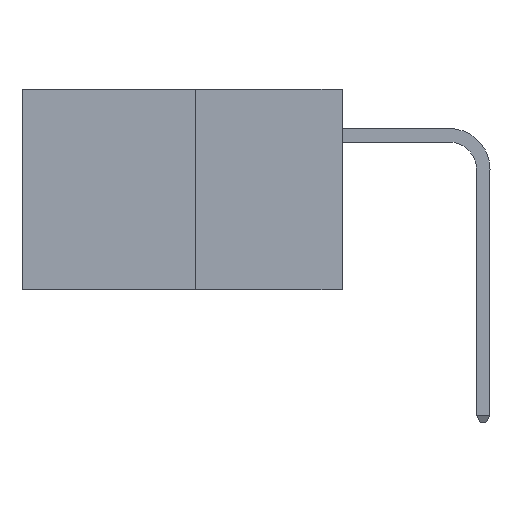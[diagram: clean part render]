
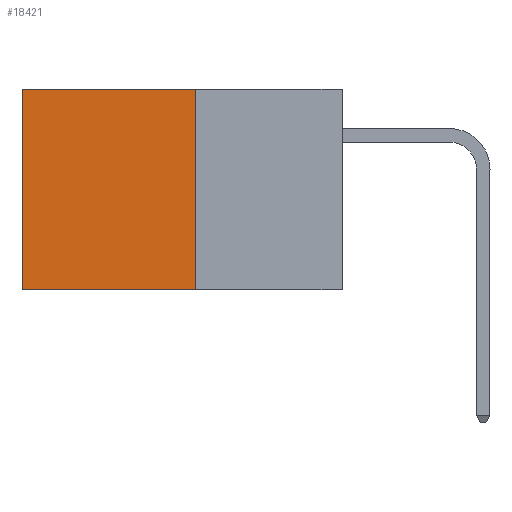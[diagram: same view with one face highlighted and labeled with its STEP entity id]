
A CAD part, left-side view. The second image highlights one B-rep face of the part: STEP entity #18421.
In plain terms, the highlighted planar face has unit normal (-1, 0, 0).
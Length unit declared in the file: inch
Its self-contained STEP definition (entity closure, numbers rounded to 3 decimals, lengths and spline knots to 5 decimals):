
#2 = CARTESIAN_POINT ( 'NONE',  ( 0.277, 0.27, 0. ) ) ;
#1806 = ORIENTED_EDGE ( 'NONE', *, *, #10412, .F. ) ;
#2340 = VERTEX_POINT ( 'NONE', #5110 ) ;
#2389 = ORIENTED_EDGE ( 'NONE', *, *, #6325, .T. ) ;
#2471 = LINE ( 'NONE', #19915, #11961 ) ;
#2724 = VECTOR ( 'NONE', #14941, 39.37008 ) ;
#2807 = DIRECTION ( 'NONE',  ( 0., 1., 0. ) ) ;
#3335 = CARTESIAN_POINT ( 'NONE',  ( 0.277, 0.27, -0.37 ) ) ;
#3695 = EDGE_CURVE ( 'NONE', #2340, #19964, #2471, .T. ) ;
#3822 = VECTOR ( 'NONE', #2807, 39.37008 ) ;
#3841 = CARTESIAN_POINT ( 'NONE',  ( 0.277, 0.59, -0.37 ) ) ;
#3886 = LINE ( 'NONE', #13002, #2724 ) ;
#4412 = LINE ( 'NONE', #10218, #3822 ) ;
#4612 = VECTOR ( 'NONE', #16706, 39.37008 ) ;
#5110 = CARTESIAN_POINT ( 'NONE',  ( 0.277, 0.59, 0. ) ) ;
#6325 = EDGE_CURVE ( 'NONE', #9844, #2340, #4412, .T. ) ;
#7610 = CARTESIAN_POINT ( 'NONE',  ( 0.277, 0.27, -0.37 ) ) ;
#8582 = CARTESIAN_POINT ( 'NONE',  ( 0.277, 0.27, -0.37 ) ) ;
#9844 = VERTEX_POINT ( 'NONE', #2 ) ;
#10218 = CARTESIAN_POINT ( 'NONE',  ( 0.277, 0.27, 0. ) ) ;
#10412 = EDGE_CURVE ( 'NONE', #9844, #19948, #3886, .T. ) ;
#10553 = DIRECTION ( 'NONE',  ( 0., 0., -1. ) ) ;
#11210 = DIRECTION ( 'NONE',  ( 0., 0., -1. ) ) ;
#11961 = VECTOR ( 'NONE', #11210, 39.37008 ) ;
#12518 = EDGE_CURVE ( 'NONE', #19948, #19964, #23747, .T. ) ;
#13002 = CARTESIAN_POINT ( 'NONE',  ( 0.277, 0.27, -0.37 ) ) ;
#14941 = DIRECTION ( 'NONE',  ( 0., 0., -1. ) ) ;
#16452 = ORIENTED_EDGE ( 'NONE', *, *, #3695, .T. ) ;
#16706 = DIRECTION ( 'NONE',  ( 0., 1., 0. ) ) ;
#18421 = ADVANCED_FACE ( 'NONE', ( #18717 ), #20136, .F. ) ;
#18717 = FACE_OUTER_BOUND ( 'NONE', #21288, .T. ) ;
#19915 = CARTESIAN_POINT ( 'NONE',  ( 0.277, 0.59, -0.37 ) ) ;
#19948 = VERTEX_POINT ( 'NONE', #7610 ) ;
#19964 = VERTEX_POINT ( 'NONE', #3841 ) ;
#20032 = ORIENTED_EDGE ( 'NONE', *, *, #12518, .F. ) ;
#20136 = PLANE ( 'NONE',  #21314 ) ;
#21288 = EDGE_LOOP ( 'NONE', ( #16452, #20032, #1806, #2389 ) ) ;
#21314 = AXIS2_PLACEMENT_3D ( 'NONE', #8582, #22074, #10553 ) ;
#22074 = DIRECTION ( 'NONE',  ( 1., 0., 0. ) ) ;
#23747 = LINE ( 'NONE', #3335, #4612 ) ;
